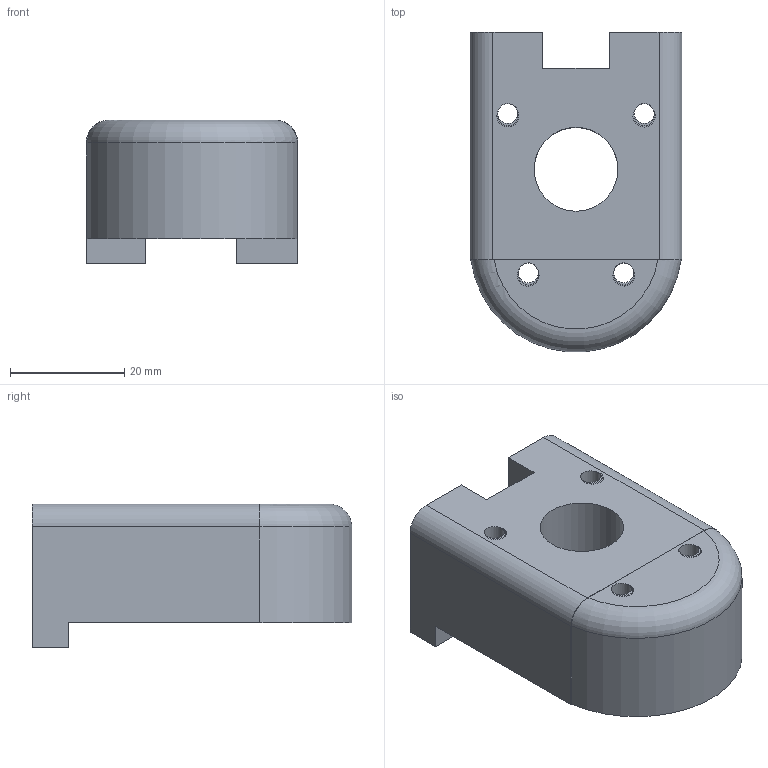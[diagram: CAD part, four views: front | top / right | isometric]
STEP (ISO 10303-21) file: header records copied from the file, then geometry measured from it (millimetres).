
FILE_DESCRIPTION(('FreeCAD Model'),'2;1');
FILE_NAME('mp-1 barrel retainer.step','2016-02-20T16:12:51',('Author'),(''), 'Open CASCADE STEP processor 6.8','FreeCAD','Unknown');
FILE_SCHEMA(('AUTOMOTIVE_DESIGN_CC2 { 1 2 10303 214 -1 1 5 4 }'));
Length unit declared in the file: millimetre
Products named in the file (1): Pocket021
Bounding box: 37.08 x 55.95 x 25.21 mm (x, y, z)
Volume: 34136.9 mm3; surface area: 9249.5 mm2
Topology: 1 solids, 2 shells, 73 faces, 213 edges, 145 vertices
Faces by surface type: plane 54, cylinder 18, torus 1
Full cylindrical faces by diameter (mm): 3.5 x4, 14.684 x3
Entity records: 6033 total; most frequent: CARTESIAN_POINT 2064, DIRECTION 695, ORIENTED_EDGE 426, PCURVE 426, DEFINITIONAL_REPRESENTATION 426, LINE 338, VECTOR 338, EDGE_CURVE 213
